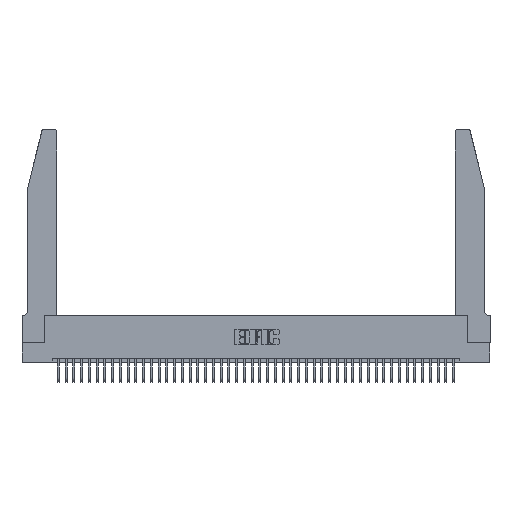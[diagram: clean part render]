
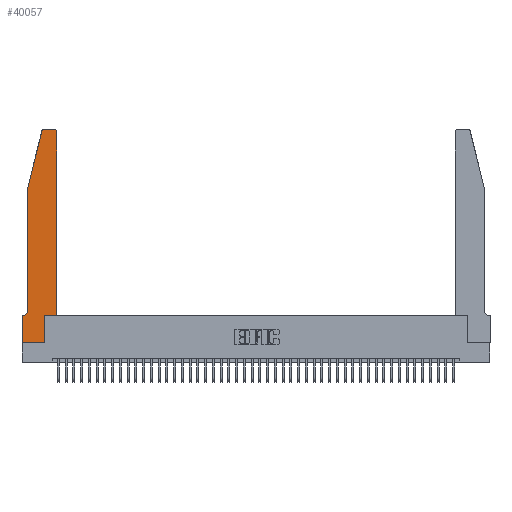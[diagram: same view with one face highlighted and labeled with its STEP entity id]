
A CAD part, top view. The second image highlights one B-rep face of the part: STEP entity #40057.
In plain terms, the highlighted planar face has unit normal (0, 0, 1).
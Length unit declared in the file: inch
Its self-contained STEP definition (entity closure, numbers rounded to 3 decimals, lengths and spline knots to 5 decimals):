
#39 = VECTOR ( 'NONE', #30353, 39.37008 ) ;
#521 = DIRECTION ( 'NONE',  ( 1., 0., 0. ) ) ;
#584 = VERTEX_POINT ( 'NONE', #28381 ) ;
#647 = CARTESIAN_POINT ( 'NONE',  ( 0.0755, 2., 0.37 ) ) ;
#1243 = VERTEX_POINT ( 'NONE', #12533 ) ;
#1782 = VERTEX_POINT ( 'NONE', #38885 ) ;
#1975 = VECTOR ( 'NONE', #9871, 39.37008 ) ;
#2437 = EDGE_CURVE ( 'NONE', #24125, #25018, #34961, .T. ) ;
#2937 = CARTESIAN_POINT ( 'NONE',  ( 0.0755, 0.35, 0.37 ) ) ;
#3103 = CARTESIAN_POINT ( 'NONE',  ( 0.4505, 0.35, 0.37 ) ) ;
#3235 = AXIS2_PLACEMENT_3D ( 'NONE', #25647, #5925, #28932 ) ;
#3960 = ORIENTED_EDGE ( 'NONE', *, *, #9942, .T. ) ;
#4040 = CARTESIAN_POINT ( 'NONE',  ( 0., 0., 0.37 ) ) ;
#4517 = LINE ( 'NONE', #11106, #28708 ) ;
#5225 = EDGE_CURVE ( 'NONE', #31022, #26641, #7443, .T. ) ;
#5361 = EDGE_CURVE ( 'NONE', #1782, #9115, #26471, .T. ) ;
#5499 = CARTESIAN_POINT ( 'NONE',  ( 0.0755, 2., 0.37 ) ) ;
#5670 = PLANE ( 'NONE',  #39992 ) ;
#5803 = DIRECTION ( 'NONE',  ( 0., 0., 1. ) ) ;
#5925 = DIRECTION ( 'NONE',  ( 0., 0., 1. ) ) ;
#6875 = VERTEX_POINT ( 'NONE', #18543 ) ;
#7356 = VECTOR ( 'NONE', #24181, 39.37008 ) ;
#7443 = CIRCLE ( 'NONE', #17343, 0.03 ) ;
#9115 = VERTEX_POINT ( 'NONE', #40469 ) ;
#9126 = VERTEX_POINT ( 'NONE', #27432 ) ;
#9871 = DIRECTION ( 'NONE',  ( 1., 0., 0. ) ) ;
#9942 = EDGE_CURVE ( 'NONE', #32170, #584, #35391, .T. ) ;
#10316 = EDGE_CURVE ( 'NONE', #9126, #27365, #19738, .T. ) ;
#10409 = CARTESIAN_POINT ( 'NONE',  ( 0., 0., 0.37 ) ) ;
#10485 = LINE ( 'NONE', #11123, #7356 ) ;
#11106 = CARTESIAN_POINT ( 'NONE',  ( 0.2605, 2.75, 0.37 ) ) ;
#11123 = CARTESIAN_POINT ( 'NONE',  ( 0.2865, 0.35, 0.37 ) ) ;
#12320 = DIRECTION ( 'NONE',  ( 0., 0., -1. ) ) ;
#12533 = CARTESIAN_POINT ( 'NONE',  ( 0.0055, 0.35, 0.37 ) ) ;
#13364 = ORIENTED_EDGE ( 'NONE', *, *, #37893, .T. ) ;
#13487 = VECTOR ( 'NONE', #42139, 39.37008 ) ;
#13876 = VECTOR ( 'NONE', #521, 39.37008 ) ;
#14816 = VECTOR ( 'NONE', #31819, 39.37008 ) ;
#14894 = LINE ( 'NONE', #10409, #13876 ) ;
#15011 = DIRECTION ( 'NONE',  ( 0., 0., 1. ) ) ;
#15703 = AXIS2_PLACEMENT_3D ( 'NONE', #31986, #12320, #35298 ) ;
#16190 = EDGE_CURVE ( 'NONE', #6875, #24125, #10485, .T. ) ;
#16760 = LINE ( 'NONE', #2937, #41863 ) ;
#17250 = ORIENTED_EDGE ( 'NONE', *, *, #23717, .T. ) ;
#17343 = AXIS2_PLACEMENT_3D ( 'NONE', #34689, #15011, #37956 ) ;
#17394 = CARTESIAN_POINT ( 'NONE',  ( 0.4205, 2.75, 0.37 ) ) ;
#18543 = CARTESIAN_POINT ( 'NONE',  ( 0.2865, 0., 0.37 ) ) ;
#18948 = CARTESIAN_POINT ( 'NONE',  ( 0., 0.35, 0.37 ) ) ;
#19278 = ORIENTED_EDGE ( 'NONE', *, *, #16190, .T. ) ;
#19738 = LINE ( 'NONE', #4040, #39 ) ;
#20412 = ORIENTED_EDGE ( 'NONE', *, *, #2437, .T. ) ;
#20452 = DIRECTION ( 'NONE',  ( -0.239, -0.971, 0. ) ) ;
#20926 = CARTESIAN_POINT ( 'NONE',  ( 0., 0., 0.37 ) ) ;
#22265 = EDGE_CURVE ( 'NONE', #584, #1243, #35188, .T. ) ;
#22670 = CARTESIAN_POINT ( 'NONE',  ( 0.4505, 0.35, 0.37 ) ) ;
#23255 = ORIENTED_EDGE ( 'NONE', *, *, #5225, .T. ) ;
#23663 = ORIENTED_EDGE ( 'NONE', *, *, #25851, .T. ) ;
#23717 = EDGE_CURVE ( 'NONE', #25018, #31022, #31985, .T. ) ;
#24100 = VECTOR ( 'NONE', #20452, 39.37008 ) ;
#24125 = VERTEX_POINT ( 'NONE', #37815 ) ;
#24181 = DIRECTION ( 'NONE',  ( 0., 1., 0. ) ) ;
#25018 = VERTEX_POINT ( 'NONE', #3103 ) ;
#25647 = CARTESIAN_POINT ( 'NONE',  ( 0.284, 2.72, 0.37 ) ) ;
#25769 = ORIENTED_EDGE ( 'NONE', *, *, #37999, .T. ) ;
#25789 = ORIENTED_EDGE ( 'NONE', *, *, #5361, .T. ) ;
#25851 = EDGE_CURVE ( 'NONE', #27365, #6875, #14894, .T. ) ;
#26471 = CIRCLE ( 'NONE', #3235, 0.03 ) ;
#26641 = VERTEX_POINT ( 'NONE', #17394 ) ;
#26643 = ORIENTED_EDGE ( 'NONE', *, *, #34245, .T. ) ;
#27365 = VERTEX_POINT ( 'NONE', #20926 ) ;
#27432 = CARTESIAN_POINT ( 'NONE',  ( 0., 0.35, 0.37 ) ) ;
#28381 = CARTESIAN_POINT ( 'NONE',  ( 0.0755, 0.42, 0.37 ) ) ;
#28708 = VECTOR ( 'NONE', #40623, 39.37008 ) ;
#28830 = DIRECTION ( 'NONE',  ( 1., 0., 0. ) ) ;
#28932 = DIRECTION ( 'NONE',  ( 1., 0., 0. ) ) ;
#28969 = ORIENTED_EDGE ( 'NONE', *, *, #22265, .T. ) ;
#29536 = CARTESIAN_POINT ( 'NONE',  ( 0.4505, 0.35, 0.37 ) ) ;
#30353 = DIRECTION ( 'NONE',  ( 0., -1., 0. ) ) ;
#31022 = VERTEX_POINT ( 'NONE', #34433 ) ;
#31819 = DIRECTION ( 'NONE',  ( 0., -1., 0. ) ) ;
#31985 = LINE ( 'NONE', #22670, #13487 ) ;
#31986 = CARTESIAN_POINT ( 'NONE',  ( 0.0055, 0.42, 0.37 ) ) ;
#32170 = VERTEX_POINT ( 'NONE', #35338 ) ;
#32845 = LINE ( 'NONE', #647, #24100 ) ;
#34245 = EDGE_CURVE ( 'NONE', #1243, #9126, #16760, .T. ) ;
#34433 = CARTESIAN_POINT ( 'NONE',  ( 0.4505, 2.72, 0.37 ) ) ;
#34689 = CARTESIAN_POINT ( 'NONE',  ( 0.4205, 2.72, 0.37 ) ) ;
#34961 = LINE ( 'NONE', #29536, #1975 ) ;
#35188 = CIRCLE ( 'NONE', #15703, 0.07 ) ;
#35298 = DIRECTION ( 'NONE',  ( -1., 0., 0. ) ) ;
#35338 = CARTESIAN_POINT ( 'NONE',  ( 0.0755, 2., 0.37 ) ) ;
#35391 = LINE ( 'NONE', #5499, #14816 ) ;
#35989 = EDGE_LOOP ( 'NONE', ( #25769, #25789, #13364, #3960, #28969, #26643, #36834, #23663, #19278, #20412, #17250, #23255 ) ) ;
#36834 = ORIENTED_EDGE ( 'NONE', *, *, #10316, .T. ) ;
#37815 = CARTESIAN_POINT ( 'NONE',  ( 0.2865, 0.35, 0.37 ) ) ;
#37893 = EDGE_CURVE ( 'NONE', #9115, #32170, #32845, .T. ) ;
#37956 = DIRECTION ( 'NONE',  ( 1., 0., 0. ) ) ;
#37999 = EDGE_CURVE ( 'NONE', #26641, #1782, #4517, .T. ) ;
#38770 = FACE_OUTER_BOUND ( 'NONE', #35989, .T. ) ;
#38885 = CARTESIAN_POINT ( 'NONE',  ( 0.284, 2.75, 0.37 ) ) ;
#39023 = DIRECTION ( 'NONE',  ( -1., 0., 0. ) ) ;
#39992 = AXIS2_PLACEMENT_3D ( 'NONE', #18948, #5803, #28830 ) ;
#40057 = ADVANCED_FACE ( 'NONE', ( #38770 ), #5670, .T. ) ;
#40469 = CARTESIAN_POINT ( 'NONE',  ( 0.25487, 2.72718, 0.37 ) ) ;
#40623 = DIRECTION ( 'NONE',  ( -1., 0., 0. ) ) ;
#41863 = VECTOR ( 'NONE', #39023, 39.37008 ) ;
#42139 = DIRECTION ( 'NONE',  ( 0., 1., 0. ) ) ;
